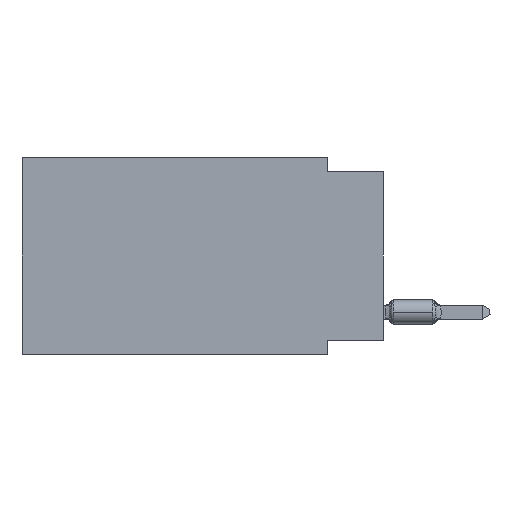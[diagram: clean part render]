
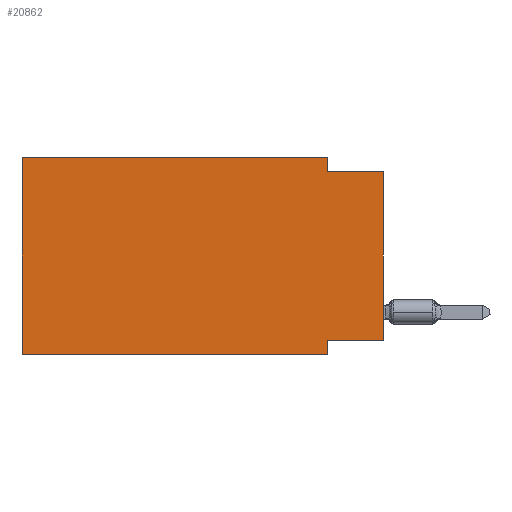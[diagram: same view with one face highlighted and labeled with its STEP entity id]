
A CAD part, left-side view. The second image highlights one B-rep face of the part: STEP entity #20862.
In plain terms, the highlighted planar face has unit normal (-1, 0, 0).
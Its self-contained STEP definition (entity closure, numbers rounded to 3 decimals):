
#467 = VERTEX_POINT ( 'NONE', #31191 ) ;
#1375 = LINE ( 'NONE', #37974, #27317 ) ;
#2245 = DIRECTION ( 'NONE',  ( 0., 0., -1. ) ) ;
#2326 = ORIENTED_EDGE ( 'NONE', *, *, #32780, .F. ) ;
#2648 = CARTESIAN_POINT ( 'NONE',  ( 0., 0., -8.255 ) ) ;
#4497 = VECTOR ( 'NONE', #36381, 1000. ) ;
#4668 = VECTOR ( 'NONE', #21501, 1000. ) ;
#5623 = CARTESIAN_POINT ( 'NONE',  ( 0., 16.383, 0. ) ) ;
#5797 = LINE ( 'NONE', #22349, #35461 ) ;
#7839 = EDGE_CURVE ( 'NONE', #31059, #28976, #9479, .T. ) ;
#9479 = LINE ( 'NONE', #22931, #4497 ) ;
#11818 = VECTOR ( 'NONE', #39910, 1000. ) ;
#11896 = ORIENTED_EDGE ( 'NONE', *, *, #18036, .F. ) ;
#12378 = PLANE ( 'NONE',  #41904 ) ;
#12455 = LINE ( 'NONE', #5623, #4668 ) ;
#14742 = CARTESIAN_POINT ( 'NONE',  ( 0., 16.383, 0. ) ) ;
#15808 = EDGE_CURVE ( 'NONE', #38307, #38639, #23784, .T. ) ;
#18036 = EDGE_CURVE ( 'NONE', #43475, #28976, #1375, .T. ) ;
#18083 = ORIENTED_EDGE ( 'NONE', *, *, #39271, .T. ) ;
#18106 = CARTESIAN_POINT ( 'NONE',  ( 0., 2.54, 0. ) ) ;
#18146 = LINE ( 'NONE', #24741, #33714 ) ;
#18794 = DIRECTION ( 'NONE',  ( 0., -1., 0. ) ) ;
#18907 = EDGE_CURVE ( 'NONE', #31333, #43475, #18146, .T. ) ;
#19478 = LINE ( 'NONE', #39545, #33606 ) ;
#19510 = VECTOR ( 'NONE', #18794, 1000. ) ;
#20862 = ADVANCED_FACE ( 'NONE', ( #38843 ), #12378, .F. ) ;
#21069 = ORIENTED_EDGE ( 'NONE', *, *, #27275, .F. ) ;
#21438 = ORIENTED_EDGE ( 'NONE', *, *, #7839, .T. ) ;
#21501 = DIRECTION ( 'NONE',  ( 0., 0., 1. ) ) ;
#21647 = DIRECTION ( 'NONE',  ( 0., 0., -1. ) ) ;
#22349 = CARTESIAN_POINT ( 'NONE',  ( 0., 0., -0.635 ) ) ;
#22931 = CARTESIAN_POINT ( 'NONE',  ( 0., 16.383, -8.89 ) ) ;
#23784 = LINE ( 'NONE', #30389, #11818 ) ;
#24741 = CARTESIAN_POINT ( 'NONE',  ( 0., 0., -8.255 ) ) ;
#24943 = DIRECTION ( 'NONE',  ( 1., 0., 0. ) ) ;
#25524 = CARTESIAN_POINT ( 'NONE',  ( 0., 2.54, -0.635 ) ) ;
#25775 = CARTESIAN_POINT ( 'NONE',  ( 0., 2.54, -8.89 ) ) ;
#26264 = ORIENTED_EDGE ( 'NONE', *, *, #18907, .F. ) ;
#27275 = EDGE_CURVE ( 'NONE', #38639, #467, #5797, .T. ) ;
#27317 = VECTOR ( 'NONE', #21647, 1000. ) ;
#28976 = VERTEX_POINT ( 'NONE', #25775 ) ;
#30195 = ORIENTED_EDGE ( 'NONE', *, *, #15808, .F. ) ;
#30389 = CARTESIAN_POINT ( 'NONE',  ( 0., 2.54, 0. ) ) ;
#31059 = VERTEX_POINT ( 'NONE', #36203 ) ;
#31191 = CARTESIAN_POINT ( 'NONE',  ( 0., 0., -0.635 ) ) ;
#31333 = VERTEX_POINT ( 'NONE', #2648 ) ;
#31591 = DIRECTION ( 'NONE',  ( 0., 1., 0. ) ) ;
#32654 = CARTESIAN_POINT ( 'NONE',  ( 0., 16.383, 0. ) ) ;
#32780 = EDGE_CURVE ( 'NONE', #31059, #38665, #12455, .T. ) ;
#33126 = DIRECTION ( 'NONE',  ( 0., -1., 0. ) ) ;
#33231 = EDGE_CURVE ( 'NONE', #38665, #38307, #35547, .T. ) ;
#33568 = DIRECTION ( 'NONE',  ( 0., 0., 1. ) ) ;
#33606 = VECTOR ( 'NONE', #33568, 1000. ) ;
#33714 = VECTOR ( 'NONE', #31591, 1000. ) ;
#35129 = CARTESIAN_POINT ( 'NONE',  ( 0., 16.383, 0. ) ) ;
#35461 = VECTOR ( 'NONE', #33126, 1000. ) ;
#35547 = LINE ( 'NONE', #35129, #19510 ) ;
#35607 = CARTESIAN_POINT ( 'NONE',  ( 0., 2.54, -8.255 ) ) ;
#36203 = CARTESIAN_POINT ( 'NONE',  ( 0., 16.383, -8.89 ) ) ;
#36381 = DIRECTION ( 'NONE',  ( 0., -1., 0. ) ) ;
#36777 = ORIENTED_EDGE ( 'NONE', *, *, #33231, .F. ) ;
#37974 = CARTESIAN_POINT ( 'NONE',  ( 0., 2.54, -8.89 ) ) ;
#38307 = VERTEX_POINT ( 'NONE', #18106 ) ;
#38639 = VERTEX_POINT ( 'NONE', #25524 ) ;
#38665 = VERTEX_POINT ( 'NONE', #14742 ) ;
#38843 = FACE_OUTER_BOUND ( 'NONE', #42444, .T. ) ;
#39271 = EDGE_CURVE ( 'NONE', #31333, #467, #19478, .T. ) ;
#39545 = CARTESIAN_POINT ( 'NONE',  ( 0., 0., 0. ) ) ;
#39910 = DIRECTION ( 'NONE',  ( 0., 0., -1. ) ) ;
#41904 = AXIS2_PLACEMENT_3D ( 'NONE', #32654, #24943, #2245 ) ;
#42444 = EDGE_LOOP ( 'NONE', ( #18083, #21069, #30195, #36777, #2326, #21438, #11896, #26264 ) ) ;
#43475 = VERTEX_POINT ( 'NONE', #35607 ) ;
